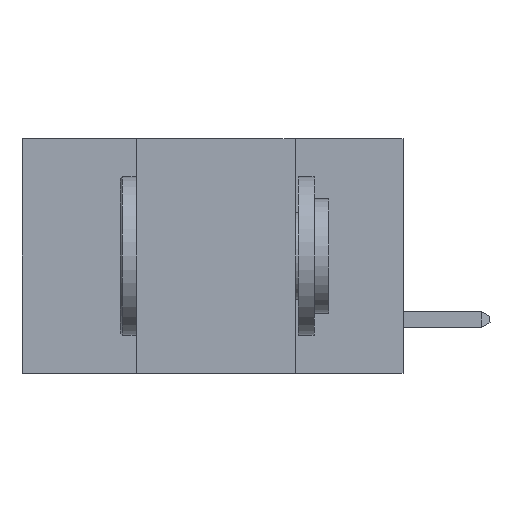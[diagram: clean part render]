
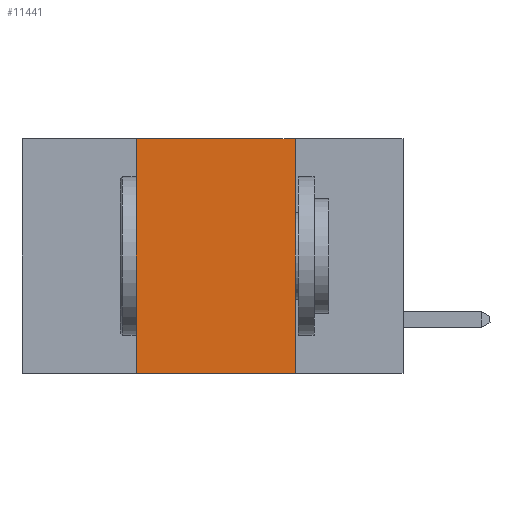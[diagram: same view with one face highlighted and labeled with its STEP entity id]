
A CAD part, left-side view. The second image highlights one B-rep face of the part: STEP entity #11441.
In plain terms, the highlighted planar face has unit normal (-1, 0, 0).
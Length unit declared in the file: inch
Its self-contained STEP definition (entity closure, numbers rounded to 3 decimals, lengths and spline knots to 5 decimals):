
#199 = CARTESIAN_POINT ( 'NONE',  ( 0., 0.42, 0. ) ) ;
#1807 = VERTEX_POINT ( 'NONE', #23253 ) ;
#2361 = EDGE_LOOP ( 'NONE', ( #22462, #8712, #17148, #21813 ) ) ;
#2656 = PLANE ( 'NONE',  #12108 ) ;
#2677 = DIRECTION ( 'NONE',  ( 0., 0., 1. ) ) ;
#3404 = VERTEX_POINT ( 'NONE', #27545 ) ;
#7349 = DIRECTION ( 'NONE',  ( 0., 0., -1. ) ) ;
#8712 = ORIENTED_EDGE ( 'NONE', *, *, #22393, .F. ) ;
#9918 = LINE ( 'NONE', #19180, #21488 ) ;
#9943 = DIRECTION ( 'NONE',  ( 0., -1., 0. ) ) ;
#9980 = DIRECTION ( 'NONE',  ( 0., -1., 0. ) ) ;
#11441 = ADVANCED_FACE ( 'NONE', ( #27753 ), #2656, .F. ) ;
#11799 = LINE ( 'NONE', #19154, #17223 ) ;
#12108 = AXIS2_PLACEMENT_3D ( 'NONE', #16647, #21249, #7349 ) ;
#13101 = EDGE_CURVE ( 'NONE', #29109, #1807, #19521, .T. ) ;
#14046 = VECTOR ( 'NONE', #24880, 39.37008 ) ;
#16487 = CARTESIAN_POINT ( 'NONE',  ( 0., 0.42, -0.37 ) ) ;
#16647 = CARTESIAN_POINT ( 'NONE',  ( 0., 0.6, 0. ) ) ;
#17148 = ORIENTED_EDGE ( 'NONE', *, *, #13101, .F. ) ;
#17223 = VECTOR ( 'NONE', #9943, 39.37008 ) ;
#18018 = CARTESIAN_POINT ( 'NONE',  ( 0., 0.17, 0. ) ) ;
#18807 = VECTOR ( 'NONE', #2677, 39.37008 ) ;
#19098 = EDGE_CURVE ( 'NONE', #3404, #20289, #20135, .T. ) ;
#19154 = CARTESIAN_POINT ( 'NONE',  ( 0., 0.6, -0.37 ) ) ;
#19180 = CARTESIAN_POINT ( 'NONE',  ( 0., 0.6, 0. ) ) ;
#19521 = LINE ( 'NONE', #199, #18807 ) ;
#20051 = EDGE_CURVE ( 'NONE', #29109, #20289, #11799, .T. ) ;
#20135 = LINE ( 'NONE', #18018, #14046 ) ;
#20289 = VERTEX_POINT ( 'NONE', #29266 ) ;
#21249 = DIRECTION ( 'NONE',  ( 1., 0., 0. ) ) ;
#21488 = VECTOR ( 'NONE', #9980, 39.37008 ) ;
#21813 = ORIENTED_EDGE ( 'NONE', *, *, #20051, .T. ) ;
#22393 = EDGE_CURVE ( 'NONE', #1807, #3404, #9918, .T. ) ;
#22462 = ORIENTED_EDGE ( 'NONE', *, *, #19098, .F. ) ;
#23253 = CARTESIAN_POINT ( 'NONE',  ( 0., 0.42, 0. ) ) ;
#24880 = DIRECTION ( 'NONE',  ( 0., 0., -1. ) ) ;
#27545 = CARTESIAN_POINT ( 'NONE',  ( 0., 0.17, 0. ) ) ;
#27753 = FACE_OUTER_BOUND ( 'NONE', #2361, .T. ) ;
#29109 = VERTEX_POINT ( 'NONE', #16487 ) ;
#29266 = CARTESIAN_POINT ( 'NONE',  ( 0., 0.17, -0.37 ) ) ;
